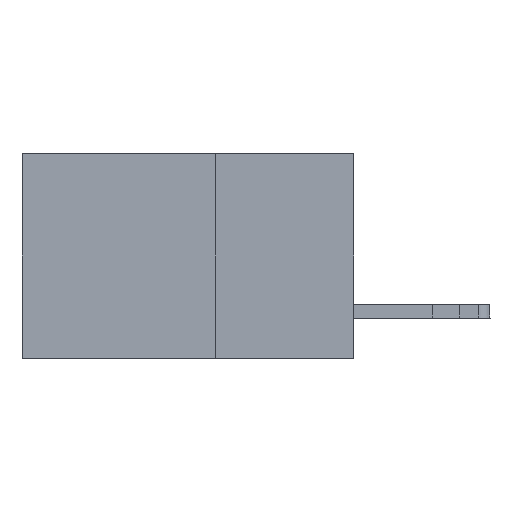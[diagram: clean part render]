
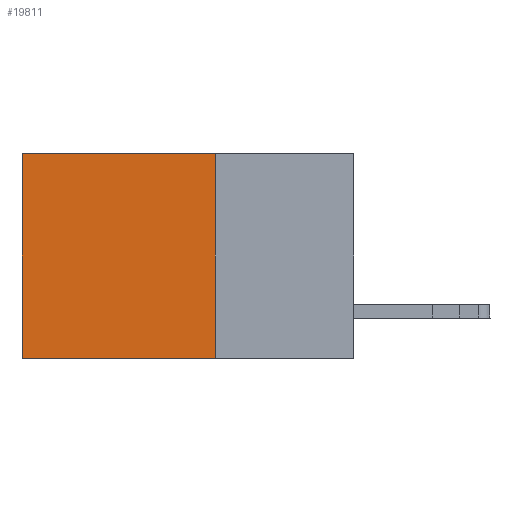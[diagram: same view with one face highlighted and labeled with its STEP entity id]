
A CAD part, left-side view. The second image highlights one B-rep face of the part: STEP entity #19811.
In plain terms, the highlighted planar face has unit normal (-1, 0, 0).
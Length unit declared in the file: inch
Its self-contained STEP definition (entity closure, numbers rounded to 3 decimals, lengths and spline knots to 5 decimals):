
#1502 = VERTEX_POINT ( 'NONE', #17546 ) ;
#1569 = FACE_OUTER_BOUND ( 'NONE', #13048, .T. ) ;
#1888 = VERTEX_POINT ( 'NONE', #16187 ) ;
#2372 = CARTESIAN_POINT ( 'NONE',  ( 0.2875, 0.6, 0. ) ) ;
#2539 = VECTOR ( 'NONE', #18416, 39.37008 ) ;
#3959 = EDGE_CURVE ( 'NONE', #8712, #1888, #19640, .T. ) ;
#4598 = DIRECTION ( 'NONE',  ( 0., 0., -1. ) ) ;
#5145 = EDGE_CURVE ( 'NONE', #1502, #11755, #19601, .T. ) ;
#7122 = ORIENTED_EDGE ( 'NONE', *, *, #5145, .F. ) ;
#7175 = AXIS2_PLACEMENT_3D ( 'NONE', #15532, #9147, #9291 ) ;
#7633 = CARTESIAN_POINT ( 'NONE',  ( 0.2875, 0.25, 0. ) ) ;
#8712 = VERTEX_POINT ( 'NONE', #17820 ) ;
#9147 = DIRECTION ( 'NONE',  ( 1., 0., 0. ) ) ;
#9291 = DIRECTION ( 'NONE',  ( 0., 0., -1. ) ) ;
#9323 = VECTOR ( 'NONE', #20413, 39.37008 ) ;
#11755 = VERTEX_POINT ( 'NONE', #20393 ) ;
#11809 = DIRECTION ( 'NONE',  ( 0., 1., 0. ) ) ;
#11904 = LINE ( 'NONE', #2372, #2539 ) ;
#12436 = CARTESIAN_POINT ( 'NONE',  ( 0.2875, 0.25, -0.37 ) ) ;
#12486 = VECTOR ( 'NONE', #4598, 39.37008 ) ;
#12842 = ORIENTED_EDGE ( 'NONE', *, *, #3959, .T. ) ;
#13048 = EDGE_LOOP ( 'NONE', ( #13952, #7122, #15894, #12842 ) ) ;
#13248 = EDGE_CURVE ( 'NONE', #1888, #11755, #11904, .T. ) ;
#13952 = ORIENTED_EDGE ( 'NONE', *, *, #13248, .T. ) ;
#15394 = PLANE ( 'NONE',  #7175 ) ;
#15532 = CARTESIAN_POINT ( 'NONE',  ( 0.2875, 0.25, 0. ) ) ;
#15894 = ORIENTED_EDGE ( 'NONE', *, *, #17054, .F. ) ;
#16187 = CARTESIAN_POINT ( 'NONE',  ( 0.2875, 0.6, 0. ) ) ;
#16188 = LINE ( 'NONE', #7633, #12486 ) ;
#17054 = EDGE_CURVE ( 'NONE', #8712, #1502, #16188, .T. ) ;
#17195 = CARTESIAN_POINT ( 'NONE',  ( 0.2875, 0.25, 0. ) ) ;
#17546 = CARTESIAN_POINT ( 'NONE',  ( 0.2875, 0.25, -0.37 ) ) ;
#17820 = CARTESIAN_POINT ( 'NONE',  ( 0.2875, 0.25, 0. ) ) ;
#18416 = DIRECTION ( 'NONE',  ( 0., 0., -1. ) ) ;
#19601 = LINE ( 'NONE', #12436, #19849 ) ;
#19640 = LINE ( 'NONE', #17195, #9323 ) ;
#19811 = ADVANCED_FACE ( 'NONE', ( #1569 ), #15394, .F. ) ;
#19849 = VECTOR ( 'NONE', #11809, 39.37008 ) ;
#20393 = CARTESIAN_POINT ( 'NONE',  ( 0.2875, 0.6, -0.37 ) ) ;
#20413 = DIRECTION ( 'NONE',  ( 0., 1., 0. ) ) ;
